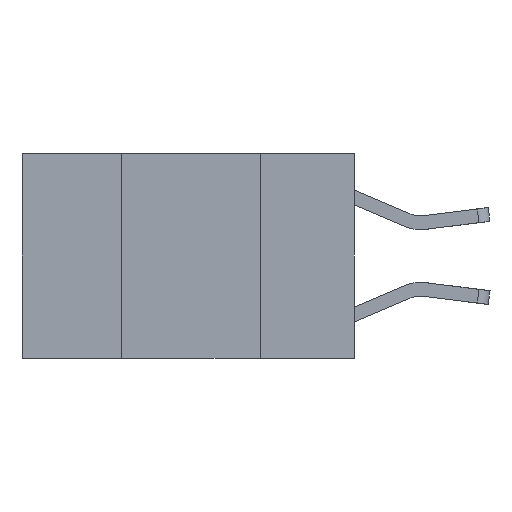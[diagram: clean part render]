
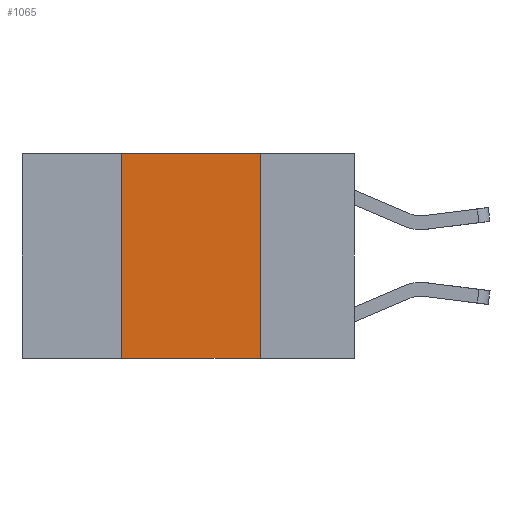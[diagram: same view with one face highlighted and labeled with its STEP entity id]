
A CAD part, left-side view. The second image highlights one B-rep face of the part: STEP entity #1065.
In plain terms, the highlighted planar face has unit normal (-1, 0, 0).
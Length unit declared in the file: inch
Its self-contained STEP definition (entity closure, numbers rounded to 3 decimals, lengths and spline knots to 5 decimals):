
#384 = ORIENTED_EDGE ( 'NONE', *, *, #8981, .F. ) ;
#518 = ORIENTED_EDGE ( 'NONE', *, *, #8018, .F. ) ;
#657 = VECTOR ( 'NONE', #2196, 39.37008 ) ;
#779 = CARTESIAN_POINT ( 'NONE',  ( 0., 0.17, -0.37 ) ) ;
#817 = CARTESIAN_POINT ( 'NONE',  ( 0., 0.17, 0. ) ) ;
#866 = DIRECTION ( 'NONE',  ( 0., 0., 1. ) ) ;
#1065 = ADVANCED_FACE ( 'NONE', ( #5028 ), #6908, .F. ) ;
#1384 = ORIENTED_EDGE ( 'NONE', *, *, #9286, .T. ) ;
#1551 = DIRECTION ( 'NONE',  ( 0., -1., 0. ) ) ;
#1569 = VERTEX_POINT ( 'NONE', #779 ) ;
#2122 = VERTEX_POINT ( 'NONE', #8052 ) ;
#2196 = DIRECTION ( 'NONE',  ( 0., -1., 0. ) ) ;
#3015 = VERTEX_POINT ( 'NONE', #7776 ) ;
#3207 = LINE ( 'NONE', #6071, #657 ) ;
#4155 = DIRECTION ( 'NONE',  ( 0., 0., -1. ) ) ;
#4170 = CARTESIAN_POINT ( 'NONE',  ( 0., 0.42, 0. ) ) ;
#4611 = VECTOR ( 'NONE', #1551, 39.37008 ) ;
#4828 = LINE ( 'NONE', #5501, #4611 ) ;
#5028 = FACE_OUTER_BOUND ( 'NONE', #6343, .T. ) ;
#5501 = CARTESIAN_POINT ( 'NONE',  ( 0., 0.6, -0.37 ) ) ;
#6071 = CARTESIAN_POINT ( 'NONE',  ( 0., 0.6, 0. ) ) ;
#6077 = AXIS2_PLACEMENT_3D ( 'NONE', #6909, #6877, #6845 ) ;
#6343 = EDGE_LOOP ( 'NONE', ( #8062, #518, #384, #1384 ) ) ;
#6445 = VERTEX_POINT ( 'NONE', #8461 ) ;
#6845 = DIRECTION ( 'NONE',  ( 0., 0., -1. ) ) ;
#6877 = DIRECTION ( 'NONE',  ( 1., 0., 0. ) ) ;
#6908 = PLANE ( 'NONE',  #6077 ) ;
#6909 = CARTESIAN_POINT ( 'NONE',  ( 0., 0.6, 0. ) ) ;
#7423 = LINE ( 'NONE', #817, #7671 ) ;
#7671 = VECTOR ( 'NONE', #4155, 39.37008 ) ;
#7776 = CARTESIAN_POINT ( 'NONE',  ( 0., 0.42, 0. ) ) ;
#8018 = EDGE_CURVE ( 'NONE', #3015, #2122, #3207, .T. ) ;
#8052 = CARTESIAN_POINT ( 'NONE',  ( 0., 0.17, 0. ) ) ;
#8062 = ORIENTED_EDGE ( 'NONE', *, *, #9386, .F. ) ;
#8461 = CARTESIAN_POINT ( 'NONE',  ( 0., 0.42, -0.37 ) ) ;
#8955 = LINE ( 'NONE', #4170, #9847 ) ;
#8981 = EDGE_CURVE ( 'NONE', #6445, #3015, #8955, .T. ) ;
#9286 = EDGE_CURVE ( 'NONE', #6445, #1569, #4828, .T. ) ;
#9386 = EDGE_CURVE ( 'NONE', #2122, #1569, #7423, .T. ) ;
#9847 = VECTOR ( 'NONE', #866, 39.37008 ) ;
